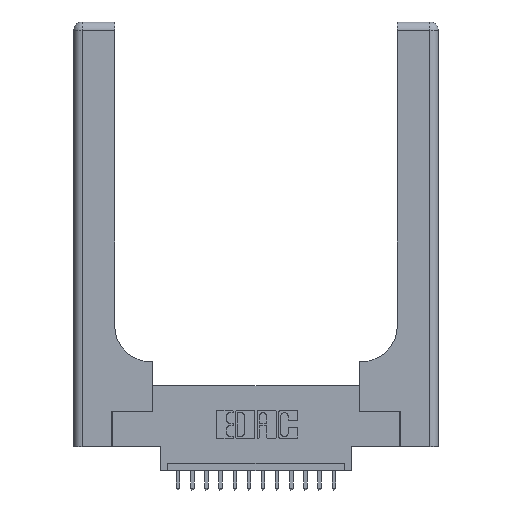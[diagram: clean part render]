
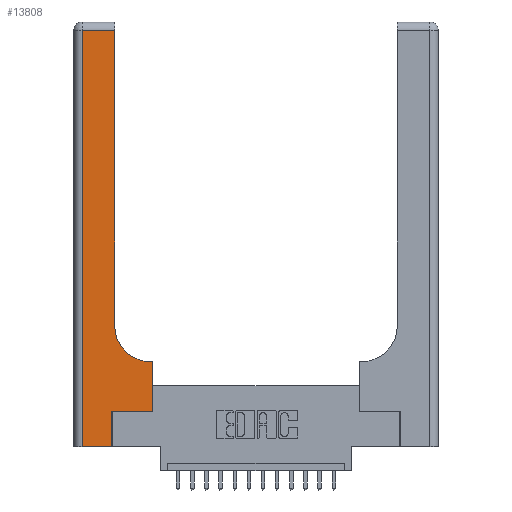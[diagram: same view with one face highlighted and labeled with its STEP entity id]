
A CAD part, top view. The second image highlights one B-rep face of the part: STEP entity #13808.
In plain terms, the highlighted planar face has unit normal (0, 0, 1).
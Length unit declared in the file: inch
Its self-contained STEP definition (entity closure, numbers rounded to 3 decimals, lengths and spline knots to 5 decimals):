
#17 = LINE ( 'NONE', #15888, #4041 ) ;
#290 = CARTESIAN_POINT ( 'NONE',  ( 0.06, 0., 0.37 ) ) ;
#348 = CARTESIAN_POINT ( 'NONE',  ( 0.269, 0., 0.37 ) ) ;
#704 = VERTEX_POINT ( 'NONE', #12035 ) ;
#1150 = EDGE_CURVE ( 'NONE', #8637, #3474, #15420, .T. ) ;
#1326 = DIRECTION ( 'NONE',  ( 0., -1., 0. ) ) ;
#1480 = CARTESIAN_POINT ( 'NONE',  ( 0., 2.94, 0.37 ) ) ;
#1544 = DIRECTION ( 'NONE',  ( -1., 0., 0. ) ) ;
#1568 = CARTESIAN_POINT ( 'NONE',  ( 0., 3., 0.37 ) ) ;
#2298 = DIRECTION ( 'NONE',  ( 0., 1., 0. ) ) ;
#2586 = VECTOR ( 'NONE', #1326, 39.37008 ) ;
#2704 = ORIENTED_EDGE ( 'NONE', *, *, #13634, .T. ) ;
#2729 = VERTEX_POINT ( 'NONE', #15016 ) ;
#3474 = VERTEX_POINT ( 'NONE', #12791 ) ;
#3894 = CARTESIAN_POINT ( 'NONE',  ( 0.2915, 3., 0.37 ) ) ;
#4041 = VECTOR ( 'NONE', #10258, 39.37008 ) ;
#4358 = VECTOR ( 'NONE', #14116, 39.37008 ) ;
#4450 = ORIENTED_EDGE ( 'NONE', *, *, #5289, .T. ) ;
#4690 = VECTOR ( 'NONE', #6744, 39.37008 ) ;
#4701 = VECTOR ( 'NONE', #8547, 39.37008 ) ;
#4874 = VERTEX_POINT ( 'NONE', #348 ) ;
#4920 = AXIS2_PLACEMENT_3D ( 'NONE', #18298, #9979, #14078 ) ;
#5289 = EDGE_CURVE ( 'NONE', #704, #8637, #16472, .T. ) ;
#5770 = ORIENTED_EDGE ( 'NONE', *, *, #13763, .T. ) ;
#5775 = VECTOR ( 'NONE', #1544, 39.37008 ) ;
#5801 = VECTOR ( 'NONE', #2298, 39.37008 ) ;
#6071 = ORIENTED_EDGE ( 'NONE', *, *, #10469, .T. ) ;
#6744 = DIRECTION ( 'NONE',  ( 1., 0., 0. ) ) ;
#6842 = ORIENTED_EDGE ( 'NONE', *, *, #12882, .T. ) ;
#6902 = LINE ( 'NONE', #8124, #5801 ) ;
#7285 = CARTESIAN_POINT ( 'NONE',  ( 0.06, 2.94, 0.37 ) ) ;
#7374 = ORIENTED_EDGE ( 'NONE', *, *, #8091, .T. ) ;
#7483 = PLANE ( 'NONE',  #17125 ) ;
#7729 = LINE ( 'NONE', #10994, #2586 ) ;
#8091 = EDGE_CURVE ( 'NONE', #8551, #11714, #7729, .T. ) ;
#8124 = CARTESIAN_POINT ( 'NONE',  ( 0.269, 0., 0.37 ) ) ;
#8545 = CARTESIAN_POINT ( 'NONE',  ( 0.5585, 0.6, 0.37 ) ) ;
#8547 = DIRECTION ( 'NONE',  ( 0., 1., 0. ) ) ;
#8551 = VERTEX_POINT ( 'NONE', #7285 ) ;
#8637 = VERTEX_POINT ( 'NONE', #8545 ) ;
#8784 = CARTESIAN_POINT ( 'NONE',  ( 0.5585, 0.25, 0.37 ) ) ;
#9335 = CARTESIAN_POINT ( 'NONE',  ( 0.2915, 2.94, 0.37 ) ) ;
#9342 = LINE ( 'NONE', #1480, #5775 ) ;
#9623 = CIRCLE ( 'NONE', #4920, 0.25 ) ;
#9979 = DIRECTION ( 'NONE',  ( 0., 0., -1. ) ) ;
#10258 = DIRECTION ( 'NONE',  ( 1., 0., 0. ) ) ;
#10449 = FACE_OUTER_BOUND ( 'NONE', #14108, .T. ) ;
#10469 = EDGE_CURVE ( 'NONE', #3474, #2729, #9623, .T. ) ;
#10797 = ORIENTED_EDGE ( 'NONE', *, *, #1150, .T. ) ;
#10994 = CARTESIAN_POINT ( 'NONE',  ( 0.06, 3., 0.37 ) ) ;
#11450 = EDGE_CURVE ( 'NONE', #2729, #11657, #15655, .T. ) ;
#11657 = VERTEX_POINT ( 'NONE', #9335 ) ;
#11714 = VERTEX_POINT ( 'NONE', #290 ) ;
#11876 = CARTESIAN_POINT ( 'NONE',  ( 0.2915, 0.6, 0.37 ) ) ;
#12035 = CARTESIAN_POINT ( 'NONE',  ( 0.5585, 0.25, 0.37 ) ) ;
#12376 = EDGE_CURVE ( 'NONE', #4874, #14953, #6902, .T. ) ;
#12791 = CARTESIAN_POINT ( 'NONE',  ( 0.5415, 0.6, 0.37 ) ) ;
#12882 = EDGE_CURVE ( 'NONE', #14953, #704, #17, .T. ) ;
#13634 = EDGE_CURVE ( 'NONE', #11714, #4874, #15984, .T. ) ;
#13763 = EDGE_CURVE ( 'NONE', #11657, #8551, #9342, .T. ) ;
#13808 = ADVANCED_FACE ( 'NONE', ( #10449 ), #7483, .F. ) ;
#14078 = DIRECTION ( 'NONE',  ( 1., 0., 0. ) ) ;
#14108 = EDGE_LOOP ( 'NONE', ( #16894, #5770, #7374, #2704, #14954, #6842, #4450, #10797, #6071 ) ) ;
#14116 = DIRECTION ( 'NONE',  ( 0., 1., 0. ) ) ;
#14308 = DIRECTION ( 'NONE',  ( 0., 0., -1. ) ) ;
#14714 = DIRECTION ( 'NONE',  ( -1., 0., 0. ) ) ;
#14953 = VERTEX_POINT ( 'NONE', #17041 ) ;
#14954 = ORIENTED_EDGE ( 'NONE', *, *, #12376, .T. ) ;
#15016 = CARTESIAN_POINT ( 'NONE',  ( 0.2915, 0.85, 0.37 ) ) ;
#15420 = LINE ( 'NONE', #11876, #17698 ) ;
#15655 = LINE ( 'NONE', #3894, #4358 ) ;
#15888 = CARTESIAN_POINT ( 'NONE',  ( 0.269, 0.25, 0.37 ) ) ;
#15984 = LINE ( 'NONE', #17782, #4690 ) ;
#16472 = LINE ( 'NONE', #8784, #4701 ) ;
#16894 = ORIENTED_EDGE ( 'NONE', *, *, #11450, .T. ) ;
#17041 = CARTESIAN_POINT ( 'NONE',  ( 0.269, 0.25, 0.37 ) ) ;
#17125 = AXIS2_PLACEMENT_3D ( 'NONE', #1568, #14308, #17253 ) ;
#17253 = DIRECTION ( 'NONE',  ( -1., 0., 0. ) ) ;
#17698 = VECTOR ( 'NONE', #14714, 39.37008 ) ;
#17782 = CARTESIAN_POINT ( 'NONE',  ( 0., 0., 0.37 ) ) ;
#18298 = CARTESIAN_POINT ( 'NONE',  ( 0.5415, 0.85, 0.37 ) ) ;
